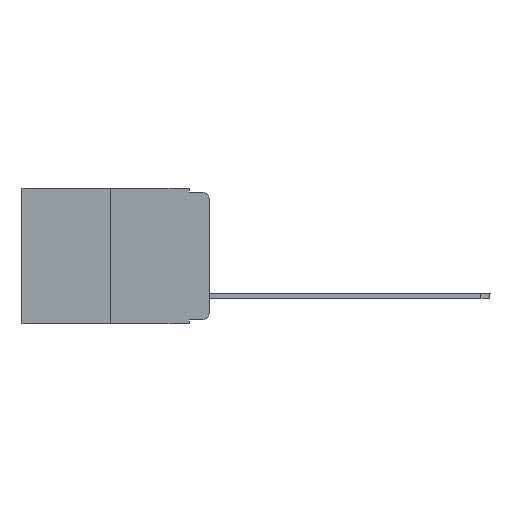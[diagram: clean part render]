
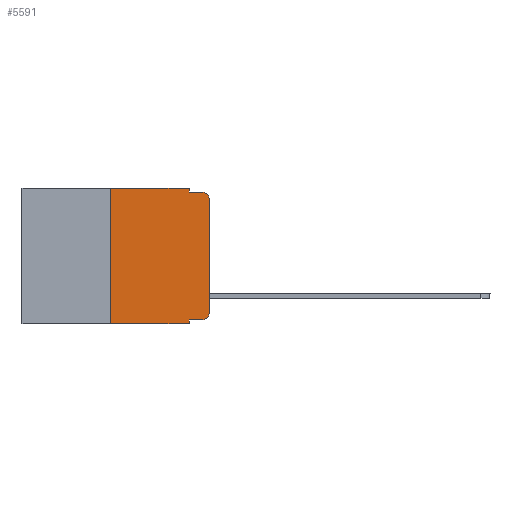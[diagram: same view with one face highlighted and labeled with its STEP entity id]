
A CAD part, left-side view. The second image highlights one B-rep face of the part: STEP entity #5591.
In plain terms, the highlighted planar face has unit normal (-1, 0, 0).
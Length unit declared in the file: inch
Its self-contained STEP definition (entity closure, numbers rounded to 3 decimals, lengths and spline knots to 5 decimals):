
#137 = CARTESIAN_POINT ( 'NONE',  ( 0., 0.051, -0.01 ) ) ;
#226 = ORIENTED_EDGE ( 'NONE', *, *, #3996, .F. ) ;
#1246 = CARTESIAN_POINT ( 'NONE',  ( 0., 0.25, 0. ) ) ;
#1293 = DIRECTION ( 'NONE',  ( 1., 0., 0. ) ) ;
#1318 = VECTOR ( 'NONE', #7149, 39.37008 ) ;
#1499 = CARTESIAN_POINT ( 'NONE',  ( 0., 0.473, 0. ) ) ;
#1585 = CARTESIAN_POINT ( 'NONE',  ( 0., 0.25, -0.343 ) ) ;
#1589 = LINE ( 'NONE', #4814, #4850 ) ;
#1657 = ORIENTED_EDGE ( 'NONE', *, *, #7604, .F. ) ;
#1919 = AXIS2_PLACEMENT_3D ( 'NONE', #13936, #6248, #8586 ) ;
#2234 = CARTESIAN_POINT ( 'NONE',  ( 0., 0., -0.313 ) ) ;
#2443 = DIRECTION ( 'NONE',  ( 0., 0., 1. ) ) ;
#2468 = VECTOR ( 'NONE', #2443, 39.37008 ) ;
#2705 = CARTESIAN_POINT ( 'NONE',  ( 0., 0.051, -0.343 ) ) ;
#2858 = ORIENTED_EDGE ( 'NONE', *, *, #6746, .T. ) ;
#2876 = CARTESIAN_POINT ( 'NONE',  ( 0., 0., 0. ) ) ;
#3004 = CARTESIAN_POINT ( 'NONE',  ( 0., 0.051, -0.333 ) ) ;
#3558 = CARTESIAN_POINT ( 'NONE',  ( 0., 0.02, -0.333 ) ) ;
#3996 = EDGE_CURVE ( 'NONE', #10693, #12331, #7794, .T. ) ;
#4123 = VERTEX_POINT ( 'NONE', #2705 ) ;
#4466 = DIRECTION ( 'NONE',  ( 0., -1., 0. ) ) ;
#4550 = EDGE_CURVE ( 'NONE', #13713, #4943, #5066, .T. ) ;
#4814 = CARTESIAN_POINT ( 'NONE',  ( 0., 0.051, -0.333 ) ) ;
#4850 = VECTOR ( 'NONE', #9920, 39.37008 ) ;
#4888 = EDGE_CURVE ( 'NONE', #12331, #7727, #8102, .T. ) ;
#4930 = ORIENTED_EDGE ( 'NONE', *, *, #12059, .F. ) ;
#4943 = VERTEX_POINT ( 'NONE', #8462 ) ;
#5066 = CIRCLE ( 'NONE', #7776, 0.02 ) ;
#5217 = EDGE_CURVE ( 'NONE', #10604, #13294, #1589, .T. ) ;
#5591 = ADVANCED_FACE ( 'NONE', ( #11218 ), #9903, .F. ) ;
#5756 = EDGE_CURVE ( 'NONE', #7592, #4123, #6084, .T. ) ;
#5803 = CARTESIAN_POINT ( 'NONE',  ( 0., 0.473, 0. ) ) ;
#5912 = ORIENTED_EDGE ( 'NONE', *, *, #4550, .T. ) ;
#5980 = EDGE_CURVE ( 'NONE', #13294, #6884, #8923, .T. ) ;
#6084 = LINE ( 'NONE', #7063, #12736 ) ;
#6122 = VECTOR ( 'NONE', #4466, 39.37008 ) ;
#6248 = DIRECTION ( 'NONE',  ( -1., 0., 0. ) ) ;
#6561 = DIRECTION ( 'NONE',  ( 0., 0., -1. ) ) ;
#6658 = VECTOR ( 'NONE', #6561, 39.37008 ) ;
#6746 = EDGE_CURVE ( 'NONE', #6884, #13713, #10301, .T. ) ;
#6831 = LINE ( 'NONE', #137, #7410 ) ;
#6884 = VERTEX_POINT ( 'NONE', #2234 ) ;
#7063 = CARTESIAN_POINT ( 'NONE',  ( 0., 0.473, -0.343 ) ) ;
#7149 = DIRECTION ( 'NONE',  ( 0., 0., -1. ) ) ;
#7410 = VECTOR ( 'NONE', #10021, 39.37008 ) ;
#7592 = VERTEX_POINT ( 'NONE', #1585 ) ;
#7604 = EDGE_CURVE ( 'NONE', #10604, #4123, #12515, .T. ) ;
#7727 = VERTEX_POINT ( 'NONE', #9769 ) ;
#7776 = AXIS2_PLACEMENT_3D ( 'NONE', #13559, #12569, #9265 ) ;
#7794 = LINE ( 'NONE', #5803, #6122 ) ;
#8102 = LINE ( 'NONE', #12398, #6658 ) ;
#8265 = DIRECTION ( 'NONE',  ( 0., 0., 1. ) ) ;
#8269 = EDGE_CURVE ( 'NONE', #7727, #4943, #6831, .T. ) ;
#8462 = CARTESIAN_POINT ( 'NONE',  ( 0., 0.02, -0.01 ) ) ;
#8577 = CARTESIAN_POINT ( 'NONE',  ( 0., 0.051, 0. ) ) ;
#8586 = DIRECTION ( 'NONE',  ( 0., 0., -1. ) ) ;
#8751 = CARTESIAN_POINT ( 'NONE',  ( 0., 0.25, 0. ) ) ;
#8875 = CARTESIAN_POINT ( 'NONE',  ( 0., 0., -0.03 ) ) ;
#8888 = LINE ( 'NONE', #8751, #2468 ) ;
#8923 = CIRCLE ( 'NONE', #1919, 0.02 ) ;
#9265 = DIRECTION ( 'NONE',  ( 0., 0., -1. ) ) ;
#9769 = CARTESIAN_POINT ( 'NONE',  ( 0., 0.051, -0.01 ) ) ;
#9903 = PLANE ( 'NONE',  #11611 ) ;
#9920 = DIRECTION ( 'NONE',  ( 0., -1., 0. ) ) ;
#10021 = DIRECTION ( 'NONE',  ( 0., -1., 0. ) ) ;
#10301 = LINE ( 'NONE', #2876, #10506 ) ;
#10506 = VECTOR ( 'NONE', #8265, 39.37008 ) ;
#10604 = VERTEX_POINT ( 'NONE', #3004 ) ;
#10693 = VERTEX_POINT ( 'NONE', #1246 ) ;
#10837 = ORIENTED_EDGE ( 'NONE', *, *, #4888, .F. ) ;
#11010 = DIRECTION ( 'NONE',  ( 0., 0., -1. ) ) ;
#11218 = FACE_OUTER_BOUND ( 'NONE', #11970, .T. ) ;
#11611 = AXIS2_PLACEMENT_3D ( 'NONE', #1499, #1293, #11010 ) ;
#11799 = ORIENTED_EDGE ( 'NONE', *, *, #5980, .T. ) ;
#11970 = EDGE_LOOP ( 'NONE', ( #2858, #5912, #12888, #10837, #226, #4930, #12262, #1657, #12891, #11799 ) ) ;
#12059 = EDGE_CURVE ( 'NONE', #7592, #10693, #8888, .T. ) ;
#12262 = ORIENTED_EDGE ( 'NONE', *, *, #5756, .T. ) ;
#12331 = VERTEX_POINT ( 'NONE', #8577 ) ;
#12398 = CARTESIAN_POINT ( 'NONE',  ( 0., 0.051, 0. ) ) ;
#12515 = LINE ( 'NONE', #12657, #1318 ) ;
#12569 = DIRECTION ( 'NONE',  ( -1., 0., 0. ) ) ;
#12657 = CARTESIAN_POINT ( 'NONE',  ( 0., 0.051, 0. ) ) ;
#12736 = VECTOR ( 'NONE', #13491, 39.37008 ) ;
#12888 = ORIENTED_EDGE ( 'NONE', *, *, #8269, .F. ) ;
#12891 = ORIENTED_EDGE ( 'NONE', *, *, #5217, .T. ) ;
#13294 = VERTEX_POINT ( 'NONE', #3558 ) ;
#13491 = DIRECTION ( 'NONE',  ( 0., -1., 0. ) ) ;
#13559 = CARTESIAN_POINT ( 'NONE',  ( 0., 0.02, -0.03 ) ) ;
#13713 = VERTEX_POINT ( 'NONE', #8875 ) ;
#13936 = CARTESIAN_POINT ( 'NONE',  ( 0., 0.02, -0.313 ) ) ;
